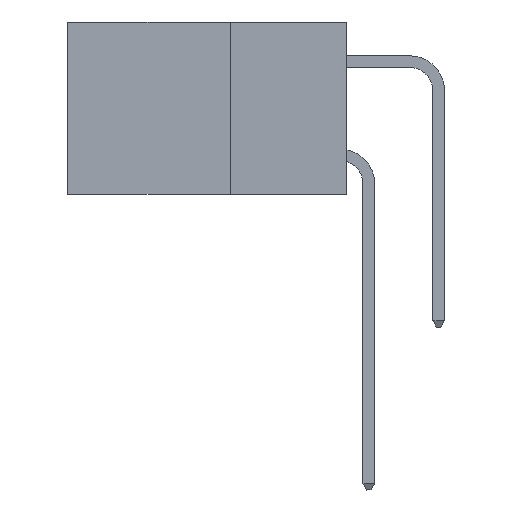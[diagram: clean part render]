
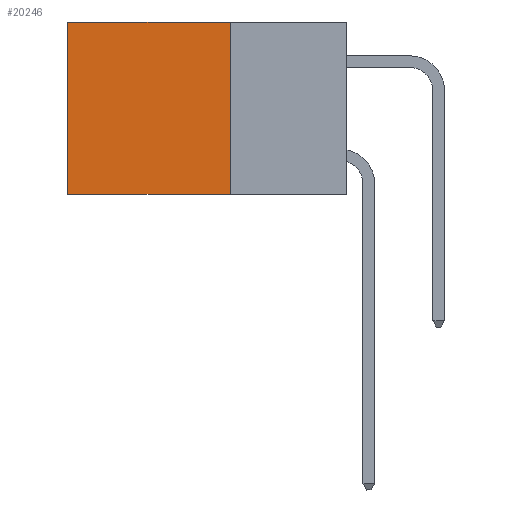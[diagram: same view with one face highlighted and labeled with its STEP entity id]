
A CAD part, left-side view. The second image highlights one B-rep face of the part: STEP entity #20246.
In plain terms, the highlighted planar face has unit normal (-1, 0, 0).
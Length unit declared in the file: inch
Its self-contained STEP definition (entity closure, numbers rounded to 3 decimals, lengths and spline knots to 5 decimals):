
#149 = VECTOR ( 'NONE', #2735, 39.37008 ) ;
#307 = DIRECTION ( 'NONE',  ( 0., 0., -1. ) ) ;
#820 = CARTESIAN_POINT ( 'NONE',  ( 0.2875, 0.25, -0.37 ) ) ;
#2071 = LINE ( 'NONE', #18269, #5995 ) ;
#2332 = PLANE ( 'NONE',  #20473 ) ;
#2372 = LINE ( 'NONE', #7230, #5984 ) ;
#2735 = DIRECTION ( 'NONE',  ( 0., 1., 0. ) ) ;
#3763 = EDGE_CURVE ( 'NONE', #10571, #15425, #2372, .T. ) ;
#4025 = EDGE_CURVE ( 'NONE', #14034, #15425, #9798, .T. ) ;
#4373 = CARTESIAN_POINT ( 'NONE',  ( 0.2875, 0.6, -0.37 ) ) ;
#4545 = ORIENTED_EDGE ( 'NONE', *, *, #3763, .T. ) ;
#4646 = VERTEX_POINT ( 'NONE', #14399 ) ;
#5984 = VECTOR ( 'NONE', #16339, 39.37008 ) ;
#5995 = VECTOR ( 'NONE', #307, 39.37008 ) ;
#6623 = LINE ( 'NONE', #13842, #149 ) ;
#7230 = CARTESIAN_POINT ( 'NONE',  ( 0.2875, 0.6, 0. ) ) ;
#7534 = FACE_OUTER_BOUND ( 'NONE', #17904, .T. ) ;
#7669 = EDGE_CURVE ( 'NONE', #4646, #14034, #2071, .T. ) ;
#7817 = ORIENTED_EDGE ( 'NONE', *, *, #7669, .F. ) ;
#7962 = ORIENTED_EDGE ( 'NONE', *, *, #11034, .T. ) ;
#8020 = DIRECTION ( 'NONE',  ( 0., 1., 0. ) ) ;
#9798 = LINE ( 'NONE', #820, #15085 ) ;
#10571 = VERTEX_POINT ( 'NONE', #18987 ) ;
#11034 = EDGE_CURVE ( 'NONE', #4646, #10571, #6623, .T. ) ;
#12666 = CARTESIAN_POINT ( 'NONE',  ( 0.2875, 0.25, -0.37 ) ) ;
#13842 = CARTESIAN_POINT ( 'NONE',  ( 0.2875, 0.25, 0. ) ) ;
#14034 = VERTEX_POINT ( 'NONE', #12666 ) ;
#14399 = CARTESIAN_POINT ( 'NONE',  ( 0.2875, 0.25, 0. ) ) ;
#14756 = DIRECTION ( 'NONE',  ( 0., 0., -1. ) ) ;
#15085 = VECTOR ( 'NONE', #8020, 39.37008 ) ;
#15101 = CARTESIAN_POINT ( 'NONE',  ( 0.2875, 0.25, 0. ) ) ;
#15425 = VERTEX_POINT ( 'NONE', #4373 ) ;
#15533 = ORIENTED_EDGE ( 'NONE', *, *, #4025, .F. ) ;
#16339 = DIRECTION ( 'NONE',  ( 0., 0., -1. ) ) ;
#17904 = EDGE_LOOP ( 'NONE', ( #4545, #15533, #7817, #7962 ) ) ;
#18269 = CARTESIAN_POINT ( 'NONE',  ( 0.2875, 0.25, 0. ) ) ;
#18987 = CARTESIAN_POINT ( 'NONE',  ( 0.2875, 0.6, 0. ) ) ;
#20246 = ADVANCED_FACE ( 'NONE', ( #7534 ), #2332, .F. ) ;
#20411 = DIRECTION ( 'NONE',  ( 1., 0., 0. ) ) ;
#20473 = AXIS2_PLACEMENT_3D ( 'NONE', #15101, #20411, #14756 ) ;
